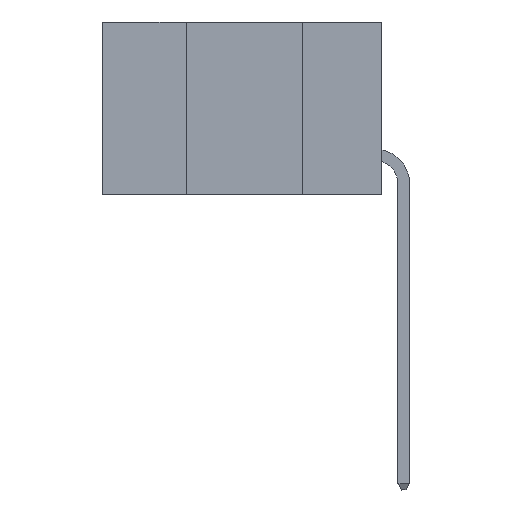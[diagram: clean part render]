
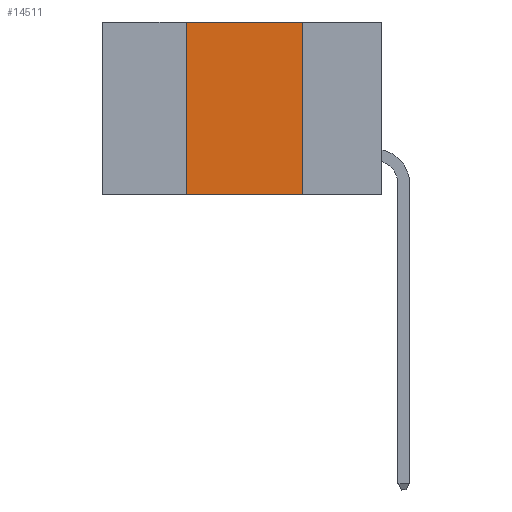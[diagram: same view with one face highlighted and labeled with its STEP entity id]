
A CAD part, left-side view. The second image highlights one B-rep face of the part: STEP entity #14511.
In plain terms, the highlighted planar face has unit normal (-1, 0, 0).
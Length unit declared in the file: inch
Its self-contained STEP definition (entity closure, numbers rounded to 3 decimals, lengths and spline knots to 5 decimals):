
#1041 = ORIENTED_EDGE ( 'NONE', *, *, #12787, .T. ) ;
#1720 = LINE ( 'NONE', #11361, #21830 ) ;
#3141 = DIRECTION ( 'NONE',  ( 0., 0., 1. ) ) ;
#4682 = ORIENTED_EDGE ( 'NONE', *, *, #18396, .F. ) ;
#10635 = CARTESIAN_POINT ( 'NONE',  ( 0., 0.17, 0. ) ) ;
#11361 = CARTESIAN_POINT ( 'NONE',  ( 0., 0.6, -0.37 ) ) ;
#12787 = EDGE_CURVE ( 'NONE', #37344, #26797, #1720, .T. ) ;
#13455 = CARTESIAN_POINT ( 'NONE',  ( 0., 0.6, 0. ) ) ;
#14511 = ADVANCED_FACE ( 'NONE', ( #40922 ), #17415, .F. ) ;
#16486 = ORIENTED_EDGE ( 'NONE', *, *, #37585, .F. ) ;
#17415 = PLANE ( 'NONE',  #20839 ) ;
#18016 = VERTEX_POINT ( 'NONE', #42035 ) ;
#18396 = EDGE_CURVE ( 'NONE', #22329, #26797, #18453, .T. ) ;
#18453 = LINE ( 'NONE', #10635, #48045 ) ;
#20839 = AXIS2_PLACEMENT_3D ( 'NONE', #43433, #21176, #47135 ) ;
#21176 = DIRECTION ( 'NONE',  ( 1., 0., 0. ) ) ;
#21830 = VECTOR ( 'NONE', #33745, 39.37008 ) ;
#22329 = VERTEX_POINT ( 'NONE', #39009 ) ;
#24014 = VECTOR ( 'NONE', #39550, 39.37008 ) ;
#26797 = VERTEX_POINT ( 'NONE', #36390 ) ;
#32585 = EDGE_CURVE ( 'NONE', #18016, #22329, #42625, .T. ) ;
#33349 = ORIENTED_EDGE ( 'NONE', *, *, #32585, .F. ) ;
#33366 = VECTOR ( 'NONE', #3141, 39.37008 ) ;
#33745 = DIRECTION ( 'NONE',  ( 0., -1., 0. ) ) ;
#34552 = LINE ( 'NONE', #44252, #33366 ) ;
#36258 = EDGE_LOOP ( 'NONE', ( #4682, #33349, #16486, #1041 ) ) ;
#36390 = CARTESIAN_POINT ( 'NONE',  ( 0., 0.17, -0.37 ) ) ;
#37344 = VERTEX_POINT ( 'NONE', #42792 ) ;
#37585 = EDGE_CURVE ( 'NONE', #37344, #18016, #34552, .T. ) ;
#39009 = CARTESIAN_POINT ( 'NONE',  ( 0., 0.17, 0. ) ) ;
#39550 = DIRECTION ( 'NONE',  ( 0., -1., 0. ) ) ;
#40232 = DIRECTION ( 'NONE',  ( 0., 0., -1. ) ) ;
#40922 = FACE_OUTER_BOUND ( 'NONE', #36258, .T. ) ;
#42035 = CARTESIAN_POINT ( 'NONE',  ( 0., 0.42, 0. ) ) ;
#42625 = LINE ( 'NONE', #13455, #24014 ) ;
#42792 = CARTESIAN_POINT ( 'NONE',  ( 0., 0.42, -0.37 ) ) ;
#43433 = CARTESIAN_POINT ( 'NONE',  ( 0., 0.6, 0. ) ) ;
#44252 = CARTESIAN_POINT ( 'NONE',  ( 0., 0.42, 0. ) ) ;
#47135 = DIRECTION ( 'NONE',  ( 0., 0., -1. ) ) ;
#48045 = VECTOR ( 'NONE', #40232, 39.37008 ) ;
